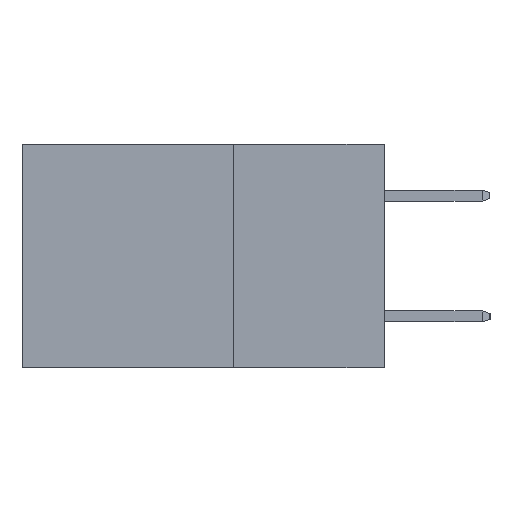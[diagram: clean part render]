
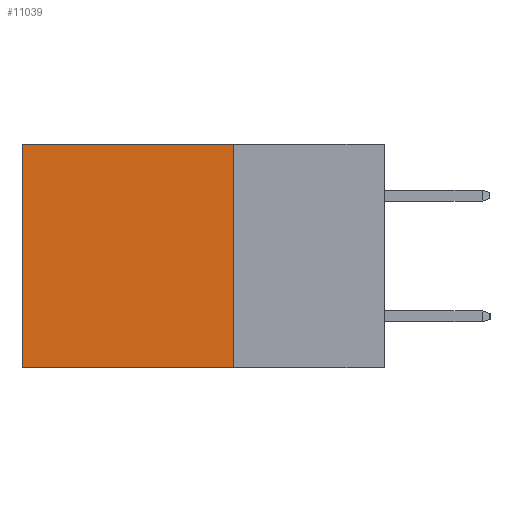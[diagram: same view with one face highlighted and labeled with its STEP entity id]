
A CAD part, left-side view. The second image highlights one B-rep face of the part: STEP entity #11039.
In plain terms, the highlighted planar face has unit normal (-1, 0, 0).
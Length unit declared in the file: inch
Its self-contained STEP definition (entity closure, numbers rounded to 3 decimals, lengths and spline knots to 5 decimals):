
#149 = LINE ( 'NONE', #7723, #14287 ) ;
#195 = CARTESIAN_POINT ( 'NONE',  ( 0.2615, 0.6, -0.37 ) ) ;
#665 = VERTEX_POINT ( 'NONE', #5886 ) ;
#1080 = ORIENTED_EDGE ( 'NONE', *, *, #2334, .F. ) ;
#1116 = EDGE_LOOP ( 'NONE', ( #11660, #5919, #1080, #13413 ) ) ;
#1313 = DIRECTION ( 'NONE',  ( 1., 0., 0. ) ) ;
#2044 = DIRECTION ( 'NONE',  ( 0., 0., -1. ) ) ;
#2327 = DIRECTION ( 'NONE',  ( 0., 1., 0. ) ) ;
#2334 = EDGE_CURVE ( 'NONE', #665, #9142, #149, .T. ) ;
#2652 = VECTOR ( 'NONE', #2327, 39.37008 ) ;
#3124 = CARTESIAN_POINT ( 'NONE',  ( 0.2615, 0.6, 0. ) ) ;
#3833 = VECTOR ( 'NONE', #8094, 39.37008 ) ;
#5884 = VECTOR ( 'NONE', #2044, 39.37008 ) ;
#5886 = CARTESIAN_POINT ( 'NONE',  ( 0.2615, 0.25, 0. ) ) ;
#5897 = VERTEX_POINT ( 'NONE', #195 ) ;
#5919 = ORIENTED_EDGE ( 'NONE', *, *, #14402, .F. ) ;
#6573 = CARTESIAN_POINT ( 'NONE',  ( 0.2615, 0.6, -0.37 ) ) ;
#6797 = LINE ( 'NONE', #10314, #3833 ) ;
#7086 = VERTEX_POINT ( 'NONE', #3124 ) ;
#7205 = CARTESIAN_POINT ( 'NONE',  ( 0.2615, 0.25, -0.37 ) ) ;
#7723 = CARTESIAN_POINT ( 'NONE',  ( 0.2615, 0.25, -0.37 ) ) ;
#7788 = EDGE_CURVE ( 'NONE', #665, #7086, #6797, .T. ) ;
#7894 = DIRECTION ( 'NONE',  ( 0., 0., -1. ) ) ;
#8016 = CARTESIAN_POINT ( 'NONE',  ( 0.2615, 0.25, -0.37 ) ) ;
#8094 = DIRECTION ( 'NONE',  ( 0., 1., 0. ) ) ;
#8576 = LINE ( 'NONE', #9001, #2652 ) ;
#9001 = CARTESIAN_POINT ( 'NONE',  ( 0.2615, 0.25, -0.37 ) ) ;
#9125 = DIRECTION ( 'NONE',  ( 0., 0., -1. ) ) ;
#9142 = VERTEX_POINT ( 'NONE', #7205 ) ;
#9406 = EDGE_CURVE ( 'NONE', #7086, #5897, #11771, .T. ) ;
#10314 = CARTESIAN_POINT ( 'NONE',  ( 0.2615, 0.25, 0. ) ) ;
#11039 = ADVANCED_FACE ( 'NONE', ( #12499 ), #12440, .F. ) ;
#11660 = ORIENTED_EDGE ( 'NONE', *, *, #9406, .T. ) ;
#11771 = LINE ( 'NONE', #6573, #5884 ) ;
#11779 = AXIS2_PLACEMENT_3D ( 'NONE', #8016, #1313, #9125 ) ;
#12440 = PLANE ( 'NONE',  #11779 ) ;
#12499 = FACE_OUTER_BOUND ( 'NONE', #1116, .T. ) ;
#13413 = ORIENTED_EDGE ( 'NONE', *, *, #7788, .T. ) ;
#14287 = VECTOR ( 'NONE', #7894, 39.37008 ) ;
#14402 = EDGE_CURVE ( 'NONE', #9142, #5897, #8576, .T. ) ;
